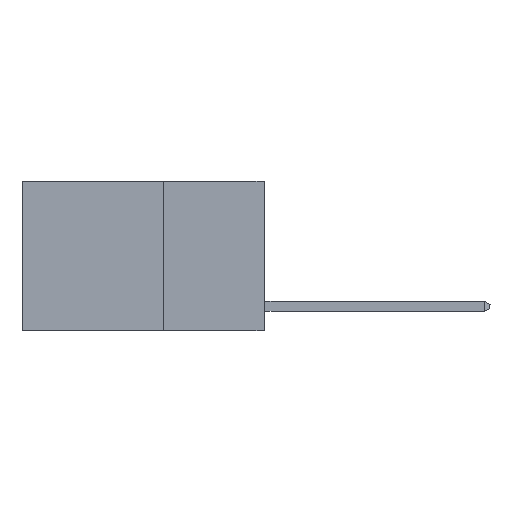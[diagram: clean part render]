
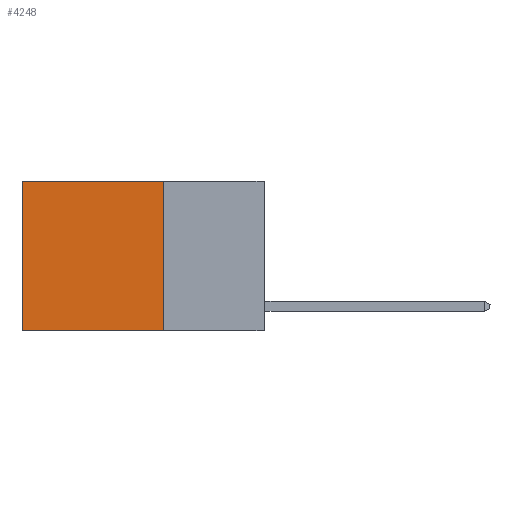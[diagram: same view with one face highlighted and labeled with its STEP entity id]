
A CAD part, left-side view. The second image highlights one B-rep face of the part: STEP entity #4248.
In plain terms, the highlighted planar face has unit normal (-1, 0, 0).
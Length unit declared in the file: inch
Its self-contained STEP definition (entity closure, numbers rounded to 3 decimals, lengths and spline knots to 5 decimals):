
#502 = LINE ( 'NONE', #10364, #5105 ) ;
#883 = DIRECTION ( 'NONE',  ( 0., 0., -1. ) ) ;
#902 = EDGE_CURVE ( 'NONE', #6337, #10458, #8159, .T. ) ;
#1656 = CARTESIAN_POINT ( 'NONE',  ( 0.2625, 0.6, 0. ) ) ;
#1913 = VERTEX_POINT ( 'NONE', #6757 ) ;
#3498 = ORIENTED_EDGE ( 'NONE', *, *, #8882, .T. ) ;
#3532 = DIRECTION ( 'NONE',  ( 0., 1., 0. ) ) ;
#3806 = AXIS2_PLACEMENT_3D ( 'NONE', #5361, #5435, #7022 ) ;
#3824 = CARTESIAN_POINT ( 'NONE',  ( 0.2625, 0.6, -0.37 ) ) ;
#4248 = ADVANCED_FACE ( 'NONE', ( #10493 ), #5815, .F. ) ;
#4395 = ORIENTED_EDGE ( 'NONE', *, *, #6156, .T. ) ;
#4845 = CARTESIAN_POINT ( 'NONE',  ( 0.2625, 0.25, 0. ) ) ;
#4936 = EDGE_CURVE ( 'NONE', #10458, #5790, #502, .T. ) ;
#5066 = ORIENTED_EDGE ( 'NONE', *, *, #902, .F. ) ;
#5105 = VECTOR ( 'NONE', #6982, 39.37008 ) ;
#5167 = CARTESIAN_POINT ( 'NONE',  ( 0.2625, 0.25, 0. ) ) ;
#5181 = VECTOR ( 'NONE', #5930, 39.37008 ) ;
#5361 = CARTESIAN_POINT ( 'NONE',  ( 0.2625, 0.25, 0. ) ) ;
#5435 = DIRECTION ( 'NONE',  ( 1., 0., 0. ) ) ;
#5790 = VERTEX_POINT ( 'NONE', #3824 ) ;
#5815 = PLANE ( 'NONE',  #3806 ) ;
#5930 = DIRECTION ( 'NONE',  ( 0., 0., -1. ) ) ;
#6156 = EDGE_CURVE ( 'NONE', #6337, #1913, #8728, .T. ) ;
#6337 = VERTEX_POINT ( 'NONE', #4845 ) ;
#6757 = CARTESIAN_POINT ( 'NONE',  ( 0.2625, 0.6, 0. ) ) ;
#6982 = DIRECTION ( 'NONE',  ( 0., 1., 0. ) ) ;
#7022 = DIRECTION ( 'NONE',  ( 0., 0., -1. ) ) ;
#7264 = EDGE_LOOP ( 'NONE', ( #3498, #8092, #5066, #4395 ) ) ;
#7511 = LINE ( 'NONE', #1656, #5181 ) ;
#7971 = CARTESIAN_POINT ( 'NONE',  ( 0.2625, 0.25, -0.37 ) ) ;
#8092 = ORIENTED_EDGE ( 'NONE', *, *, #4936, .F. ) ;
#8159 = LINE ( 'NONE', #8361, #9147 ) ;
#8361 = CARTESIAN_POINT ( 'NONE',  ( 0.2625, 0.25, 0. ) ) ;
#8512 = VECTOR ( 'NONE', #3532, 39.37008 ) ;
#8728 = LINE ( 'NONE', #5167, #8512 ) ;
#8882 = EDGE_CURVE ( 'NONE', #1913, #5790, #7511, .T. ) ;
#9147 = VECTOR ( 'NONE', #883, 39.37008 ) ;
#10364 = CARTESIAN_POINT ( 'NONE',  ( 0.2625, 0.25, -0.37 ) ) ;
#10458 = VERTEX_POINT ( 'NONE', #7971 ) ;
#10493 = FACE_OUTER_BOUND ( 'NONE', #7264, .T. ) ;
